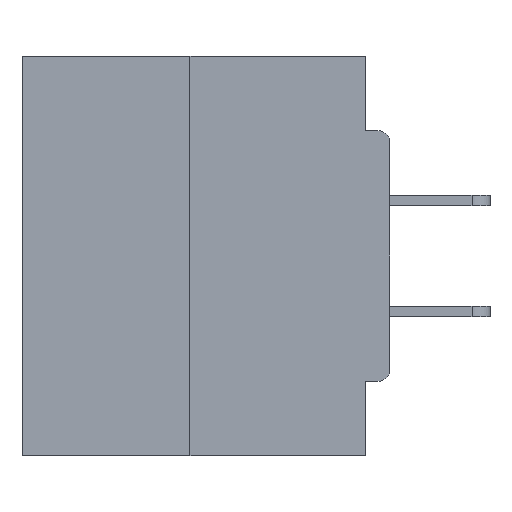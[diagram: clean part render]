
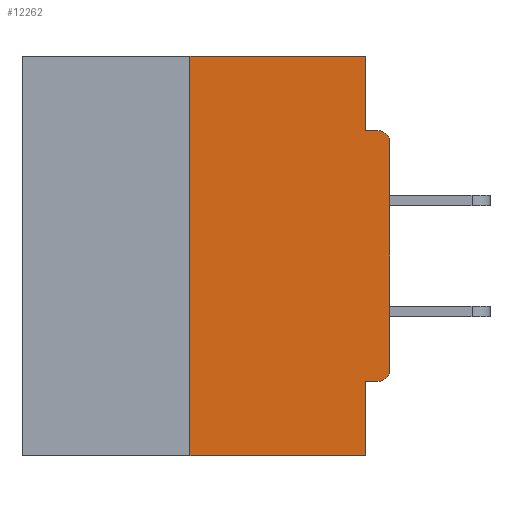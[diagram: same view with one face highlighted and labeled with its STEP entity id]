
A CAD part, left-side view. The second image highlights one B-rep face of the part: STEP entity #12262.
In plain terms, the highlighted planar face has unit normal (-1, 0, 0).
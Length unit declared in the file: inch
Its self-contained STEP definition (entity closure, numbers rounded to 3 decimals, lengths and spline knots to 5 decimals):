
#335 = DIRECTION ( 'NONE',  ( 0., 0., -1. ) ) ;
#338 = CARTESIAN_POINT ( 'NONE',  ( 0., 0.25, 0. ) ) ;
#824 = EDGE_CURVE ( 'NONE', #34174, #32605, #29523, .T. ) ;
#885 = DIRECTION ( 'NONE',  ( 1., 0., 0. ) ) ;
#1229 = CIRCLE ( 'NONE', #18179, 0.015 ) ;
#2591 = VERTEX_POINT ( 'NONE', #19568 ) ;
#2616 = CARTESIAN_POINT ( 'NONE',  ( 0., 0., -0.1085 ) ) ;
#3517 = EDGE_CURVE ( 'NONE', #25413, #34174, #11234, .T. ) ;
#3576 = CARTESIAN_POINT ( 'NONE',  ( 0., 0.46, 0. ) ) ;
#3783 = LINE ( 'NONE', #338, #5053 ) ;
#3979 = EDGE_CURVE ( 'NONE', #25413, #12390, #1229, .T. ) ;
#4016 = DIRECTION ( 'NONE',  ( 0., 0., -1. ) ) ;
#4125 = EDGE_CURVE ( 'NONE', #12390, #24931, #6495, .T. ) ;
#4798 = DIRECTION ( 'NONE',  ( 0., -1., 0. ) ) ;
#5053 = VECTOR ( 'NONE', #6090, 39.37008 ) ;
#5593 = CARTESIAN_POINT ( 'NONE',  ( 0., 0.015, -0.1085 ) ) ;
#5619 = LINE ( 'NONE', #35835, #34246 ) ;
#6090 = DIRECTION ( 'NONE',  ( 0., 0., 1. ) ) ;
#6495 = LINE ( 'NONE', #16068, #6894 ) ;
#6733 = VECTOR ( 'NONE', #4798, 39.37008 ) ;
#6761 = CIRCLE ( 'NONE', #10236, 0.015 ) ;
#6894 = VECTOR ( 'NONE', #35736, 39.37008 ) ;
#7297 = DIRECTION ( 'NONE',  ( 0., 1., 0. ) ) ;
#8003 = VERTEX_POINT ( 'NONE', #32544 ) ;
#8447 = DIRECTION ( 'NONE',  ( -1., 0., 0. ) ) ;
#8871 = PLANE ( 'NONE',  #23929 ) ;
#9152 = ORIENTED_EDGE ( 'NONE', *, *, #824, .F. ) ;
#9474 = VECTOR ( 'NONE', #27887, 39.37008 ) ;
#10236 = AXIS2_PLACEMENT_3D ( 'NONE', #5593, #8447, #335 ) ;
#10373 = CARTESIAN_POINT ( 'NONE',  ( 0., 0.015, -0.3915 ) ) ;
#10507 = CARTESIAN_POINT ( 'NONE',  ( 0., 0.031, -0.4065 ) ) ;
#10839 = VERTEX_POINT ( 'NONE', #28012 ) ;
#10885 = EDGE_CURVE ( 'NONE', #8003, #32605, #24175, .T. ) ;
#11234 = LINE ( 'NONE', #24718, #32077 ) ;
#12262 = ADVANCED_FACE ( 'NONE', ( #24961 ), #8871, .F. ) ;
#12390 = VERTEX_POINT ( 'NONE', #23746 ) ;
#13205 = EDGE_CURVE ( 'NONE', #24931, #10839, #6761, .T. ) ;
#13520 = DIRECTION ( 'NONE',  ( 0., -1., 0. ) ) ;
#14456 = DIRECTION ( 'NONE',  ( 0., 0., -1. ) ) ;
#15417 = EDGE_CURVE ( 'NONE', #8003, #28438, #3783, .T. ) ;
#16068 = CARTESIAN_POINT ( 'NONE',  ( 0., 0., 0. ) ) ;
#16243 = CARTESIAN_POINT ( 'NONE',  ( 0., 0.031, 0. ) ) ;
#16498 = EDGE_CURVE ( 'NONE', #28438, #2591, #24439, .T. ) ;
#16924 = ORIENTED_EDGE ( 'NONE', *, *, #15417, .F. ) ;
#16980 = CARTESIAN_POINT ( 'NONE',  ( 0., 0.031, -0.0935 ) ) ;
#17765 = CARTESIAN_POINT ( 'NONE',  ( 0., 0.46, 0. ) ) ;
#18179 = AXIS2_PLACEMENT_3D ( 'NONE', #10373, #24177, #18394 ) ;
#18394 = DIRECTION ( 'NONE',  ( 0., 0., -1. ) ) ;
#18440 = DIRECTION ( 'NONE',  ( 0., 0., -1. ) ) ;
#18491 = ORIENTED_EDGE ( 'NONE', *, *, #13205, .T. ) ;
#19398 = VECTOR ( 'NONE', #18440, 39.37008 ) ;
#19568 = CARTESIAN_POINT ( 'NONE',  ( 0., 0.031, 0. ) ) ;
#20619 = ORIENTED_EDGE ( 'NONE', *, *, #16498, .F. ) ;
#21233 = VECTOR ( 'NONE', #4016, 39.37008 ) ;
#22018 = CARTESIAN_POINT ( 'NONE',  ( 0., 0.015, -0.4065 ) ) ;
#22250 = ORIENTED_EDGE ( 'NONE', *, *, #4125, .T. ) ;
#23249 = CARTESIAN_POINT ( 'NONE',  ( 0., 0.031, -0.5 ) ) ;
#23497 = EDGE_LOOP ( 'NONE', ( #20619, #16924, #33235, #9152, #30635, #26586, #22250, #18491, #23597, #32846 ) ) ;
#23597 = ORIENTED_EDGE ( 'NONE', *, *, #24825, .F. ) ;
#23746 = CARTESIAN_POINT ( 'NONE',  ( 0., 0., -0.3915 ) ) ;
#23929 = AXIS2_PLACEMENT_3D ( 'NONE', #3576, #885, #14456 ) ;
#24175 = LINE ( 'NONE', #33594, #9474 ) ;
#24177 = DIRECTION ( 'NONE',  ( -1., 0., 0. ) ) ;
#24439 = LINE ( 'NONE', #17765, #6733 ) ;
#24718 = CARTESIAN_POINT ( 'NONE',  ( 0., 0., -0.4065 ) ) ;
#24825 = EDGE_CURVE ( 'NONE', #33231, #10839, #5619, .T. ) ;
#24931 = VERTEX_POINT ( 'NONE', #2616 ) ;
#24961 = FACE_OUTER_BOUND ( 'NONE', #23497, .T. ) ;
#25413 = VERTEX_POINT ( 'NONE', #22018 ) ;
#26586 = ORIENTED_EDGE ( 'NONE', *, *, #3979, .T. ) ;
#26769 = CARTESIAN_POINT ( 'NONE',  ( 0., 0.25, 0. ) ) ;
#27887 = DIRECTION ( 'NONE',  ( 0., -1., 0. ) ) ;
#27934 = CARTESIAN_POINT ( 'NONE',  ( 0., 0.031, -0.5 ) ) ;
#28012 = CARTESIAN_POINT ( 'NONE',  ( 0., 0.015, -0.0935 ) ) ;
#28438 = VERTEX_POINT ( 'NONE', #26769 ) ;
#29523 = LINE ( 'NONE', #23249, #21233 ) ;
#30635 = ORIENTED_EDGE ( 'NONE', *, *, #3517, .F. ) ;
#32077 = VECTOR ( 'NONE', #7297, 39.37008 ) ;
#32544 = CARTESIAN_POINT ( 'NONE',  ( 0., 0.25, -0.5 ) ) ;
#32605 = VERTEX_POINT ( 'NONE', #27934 ) ;
#32846 = ORIENTED_EDGE ( 'NONE', *, *, #35176, .F. ) ;
#33231 = VERTEX_POINT ( 'NONE', #16980 ) ;
#33235 = ORIENTED_EDGE ( 'NONE', *, *, #10885, .T. ) ;
#33594 = CARTESIAN_POINT ( 'NONE',  ( 0., 0.46, -0.5 ) ) ;
#34174 = VERTEX_POINT ( 'NONE', #10507 ) ;
#34175 = LINE ( 'NONE', #16243, #19398 ) ;
#34246 = VECTOR ( 'NONE', #13520, 39.37008 ) ;
#35176 = EDGE_CURVE ( 'NONE', #2591, #33231, #34175, .T. ) ;
#35736 = DIRECTION ( 'NONE',  ( 0., 0., 1. ) ) ;
#35835 = CARTESIAN_POINT ( 'NONE',  ( 0., 0., -0.0935 ) ) ;
